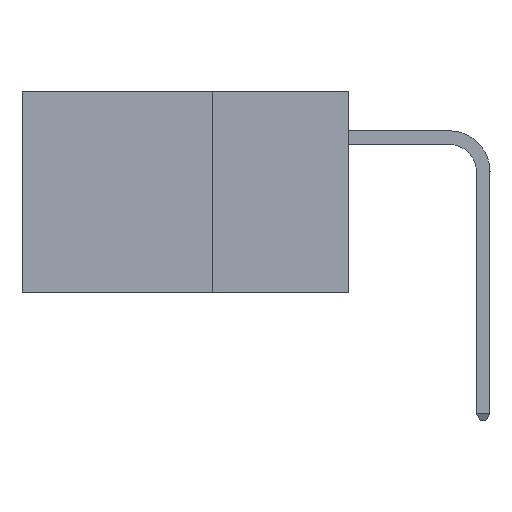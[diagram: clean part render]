
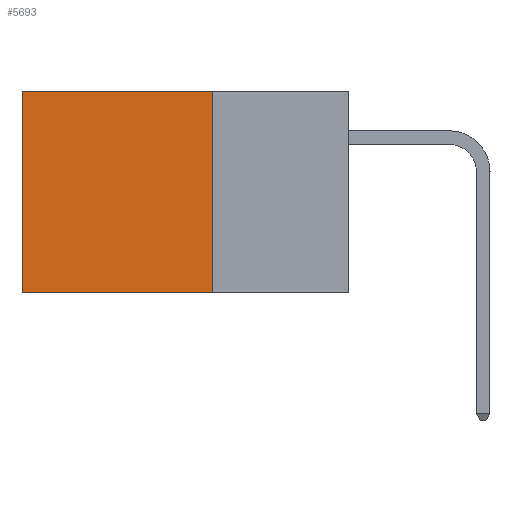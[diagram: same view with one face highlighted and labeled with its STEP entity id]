
A CAD part, left-side view. The second image highlights one B-rep face of the part: STEP entity #5693.
In plain terms, the highlighted planar face has unit normal (-1, 0, 0).
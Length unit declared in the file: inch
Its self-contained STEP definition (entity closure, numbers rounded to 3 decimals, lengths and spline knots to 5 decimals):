
#343 = CARTESIAN_POINT ( 'NONE',  ( 0.2875, 0.6, 0. ) ) ;
#838 = CARTESIAN_POINT ( 'NONE',  ( 0.2875, 0.25, 0. ) ) ;
#936 = VERTEX_POINT ( 'NONE', #838 ) ;
#1129 = CARTESIAN_POINT ( 'NONE',  ( 0.2875, 0.25, 0. ) ) ;
#1438 = VECTOR ( 'NONE', #6773, 39.37008 ) ;
#1452 = LINE ( 'NONE', #343, #1438 ) ;
#1679 = ORIENTED_EDGE ( 'NONE', *, *, #2460, .T. ) ;
#1755 = VERTEX_POINT ( 'NONE', #6042 ) ;
#2188 = VECTOR ( 'NONE', #8841, 39.37008 ) ;
#2299 = DIRECTION ( 'NONE',  ( 1., 0., 0. ) ) ;
#2347 = LINE ( 'NONE', #3185, #2188 ) ;
#2460 = EDGE_CURVE ( 'NONE', #7918, #2671, #1452, .T. ) ;
#2671 = VERTEX_POINT ( 'NONE', #3057 ) ;
#3057 = CARTESIAN_POINT ( 'NONE',  ( 0.2875, 0.6, -0.37 ) ) ;
#3185 = CARTESIAN_POINT ( 'NONE',  ( 0.2875, 0.25, 0. ) ) ;
#4538 = CARTESIAN_POINT ( 'NONE',  ( 0.2875, 0.25, -0.37 ) ) ;
#4668 = DIRECTION ( 'NONE',  ( 0., 1., 0. ) ) ;
#5259 = EDGE_CURVE ( 'NONE', #1755, #2671, #10292, .T. ) ;
#5519 = ORIENTED_EDGE ( 'NONE', *, *, #10080, .T. ) ;
#5693 = ADVANCED_FACE ( 'NONE', ( #10053 ), #7391, .F. ) ;
#6042 = CARTESIAN_POINT ( 'NONE',  ( 0.2875, 0.25, -0.37 ) ) ;
#6160 = ORIENTED_EDGE ( 'NONE', *, *, #11173, .F. ) ;
#6256 = ORIENTED_EDGE ( 'NONE', *, *, #5259, .F. ) ;
#6773 = DIRECTION ( 'NONE',  ( 0., 0., -1. ) ) ;
#6887 = AXIS2_PLACEMENT_3D ( 'NONE', #1129, #2299, #9070 ) ;
#7391 = PLANE ( 'NONE',  #6887 ) ;
#7918 = VERTEX_POINT ( 'NONE', #10974 ) ;
#8492 = EDGE_LOOP ( 'NONE', ( #1679, #6256, #6160, #5519 ) ) ;
#8841 = DIRECTION ( 'NONE',  ( 0., 0., -1. ) ) ;
#9070 = DIRECTION ( 'NONE',  ( 0., 0., -1. ) ) ;
#9151 = CARTESIAN_POINT ( 'NONE',  ( 0.2875, 0.25, 0. ) ) ;
#9296 = VECTOR ( 'NONE', #4668, 39.37008 ) ;
#9861 = DIRECTION ( 'NONE',  ( 0., 1., 0. ) ) ;
#9916 = LINE ( 'NONE', #9151, #9296 ) ;
#10036 = VECTOR ( 'NONE', #9861, 39.37008 ) ;
#10053 = FACE_OUTER_BOUND ( 'NONE', #8492, .T. ) ;
#10080 = EDGE_CURVE ( 'NONE', #936, #7918, #9916, .T. ) ;
#10292 = LINE ( 'NONE', #4538, #10036 ) ;
#10974 = CARTESIAN_POINT ( 'NONE',  ( 0.2875, 0.6, 0. ) ) ;
#11173 = EDGE_CURVE ( 'NONE', #936, #1755, #2347, .T. ) ;
